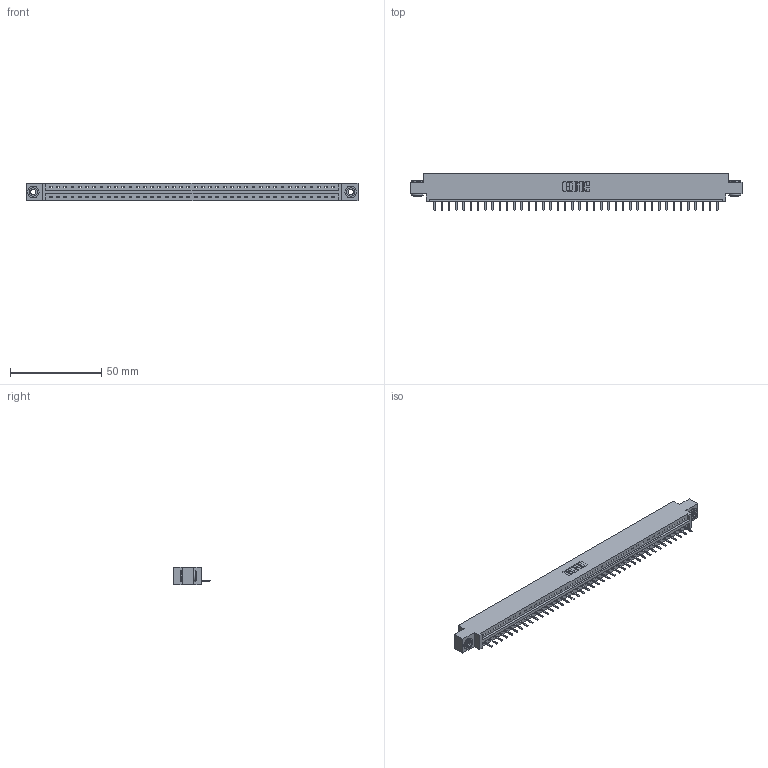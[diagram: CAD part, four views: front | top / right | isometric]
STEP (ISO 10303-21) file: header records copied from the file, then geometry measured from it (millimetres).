
FILE_DESCRIPTION (( 'STEP AP203' ), '1' );
FILE_NAME ('337-040-520-603.STEP', '2019-10-01T19:16:16', ( '' ), ( '' ), 'SwSTEP 2.0', 'SolidWorks 2016', '' );
FILE_SCHEMA (( 'CONFIG_CONTROL_DESIGN' ));
Length unit declared in the file: inch
Products named in the file (4): 345-250-002_345-250-002-102; 337-040-520-603; 337 Part_0.170 Offset - 0.156 Dia-TH; 345-292-001_345-293-120
Assembly tree (43 placements, depth 2):
  337-040-520-603
    337 Part_0.170 Offset - 0.156 Dia-TH
    345-292-001_345-293-120  x40
    345-250-002_345-250-002-102  x2
Bounding box: 181.51 x 20.02 x 9.4 mm (x, y, z)
Volume: 18626.5 mm3; surface area: 19151.6 mm2
Topology: 43 solids, 43 shells, 2796 faces, 8239 edges, 5382 vertices
Faces by surface type: plane 2004, cylinder 784, cone 8
Entity records: 30888 total; most frequent: CARTESIAN_POINT 5369, ORIENTED_EDGE 5326, DIRECTION 4545, EDGE_CURVE 2663, VECTOR 2507, LINE 2507, VERTEX_POINT 1770, AXIS2_PLACEMENT_3D 1019
